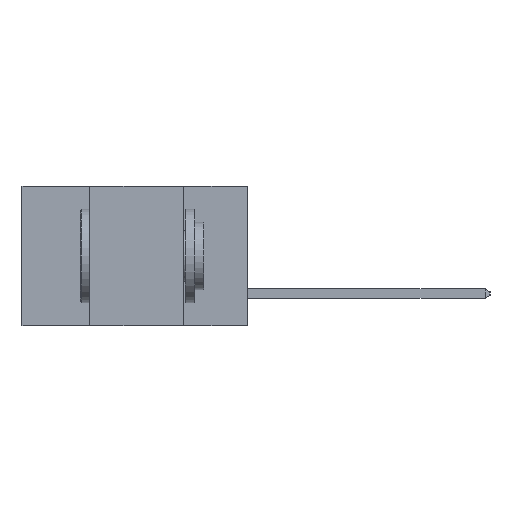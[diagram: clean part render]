
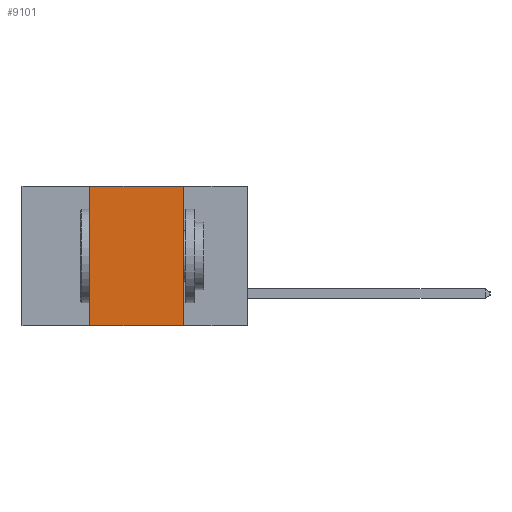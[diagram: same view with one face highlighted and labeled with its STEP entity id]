
A CAD part, left-side view. The second image highlights one B-rep face of the part: STEP entity #9101.
In plain terms, the highlighted planar face has unit normal (-1, 0, 0).
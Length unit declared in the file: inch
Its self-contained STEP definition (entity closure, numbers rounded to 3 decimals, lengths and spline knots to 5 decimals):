
#309 = ORIENTED_EDGE ( 'NONE', *, *, #2711, .F. ) ;
#329 = LINE ( 'NONE', #2050, #9382 ) ;
#607 = VERTEX_POINT ( 'NONE', #7273 ) ;
#741 = FACE_OUTER_BOUND ( 'NONE', #5385, .T. ) ;
#878 = VERTEX_POINT ( 'NONE', #5059 ) ;
#972 = VERTEX_POINT ( 'NONE', #6365 ) ;
#1459 = DIRECTION ( 'NONE',  ( 0., 0., -1. ) ) ;
#2050 = CARTESIAN_POINT ( 'NONE',  ( 0., 0.6, -0.37 ) ) ;
#2711 = EDGE_CURVE ( 'NONE', #10399, #607, #8914, .T. ) ;
#3244 = CARTESIAN_POINT ( 'NONE',  ( 0., 0.6, 0. ) ) ;
#3863 = VECTOR ( 'NONE', #5346, 39.37008 ) ;
#4142 = LINE ( 'NONE', #11102, #3863 ) ;
#4237 = DIRECTION ( 'NONE',  ( 0., -1., 0. ) ) ;
#4828 = ORIENTED_EDGE ( 'NONE', *, *, #10380, .F. ) ;
#4916 = LINE ( 'NONE', #10178, #9190 ) ;
#5059 = CARTESIAN_POINT ( 'NONE',  ( 0., 0.17, -0.37 ) ) ;
#5118 = ORIENTED_EDGE ( 'NONE', *, *, #8768, .F. ) ;
#5346 = DIRECTION ( 'NONE',  ( 0., 0., 1. ) ) ;
#5385 = EDGE_LOOP ( 'NONE', ( #4828, #309, #5118, #5409 ) ) ;
#5409 = ORIENTED_EDGE ( 'NONE', *, *, #7638, .T. ) ;
#6365 = CARTESIAN_POINT ( 'NONE',  ( 0., 0.42, -0.37 ) ) ;
#6505 = AXIS2_PLACEMENT_3D ( 'NONE', #3244, #6730, #1459 ) ;
#6649 = DIRECTION ( 'NONE',  ( 0., -1., 0. ) ) ;
#6665 = VECTOR ( 'NONE', #6649, 39.37008 ) ;
#6730 = DIRECTION ( 'NONE',  ( 1., 0., 0. ) ) ;
#7273 = CARTESIAN_POINT ( 'NONE',  ( 0., 0.17, 0. ) ) ;
#7638 = EDGE_CURVE ( 'NONE', #972, #878, #329, .T. ) ;
#8768 = EDGE_CURVE ( 'NONE', #972, #10399, #4142, .T. ) ;
#8914 = LINE ( 'NONE', #9513, #6665 ) ;
#9101 = ADVANCED_FACE ( 'NONE', ( #741 ), #9254, .F. ) ;
#9190 = VECTOR ( 'NONE', #9402, 39.37008 ) ;
#9254 = PLANE ( 'NONE',  #6505 ) ;
#9382 = VECTOR ( 'NONE', #4237, 39.37008 ) ;
#9402 = DIRECTION ( 'NONE',  ( 0., 0., -1. ) ) ;
#9436 = CARTESIAN_POINT ( 'NONE',  ( 0., 0.42, 0. ) ) ;
#9513 = CARTESIAN_POINT ( 'NONE',  ( 0., 0.6, 0. ) ) ;
#10178 = CARTESIAN_POINT ( 'NONE',  ( 0., 0.17, 0. ) ) ;
#10380 = EDGE_CURVE ( 'NONE', #607, #878, #4916, .T. ) ;
#10399 = VERTEX_POINT ( 'NONE', #9436 ) ;
#11102 = CARTESIAN_POINT ( 'NONE',  ( 0., 0.42, 0. ) ) ;
